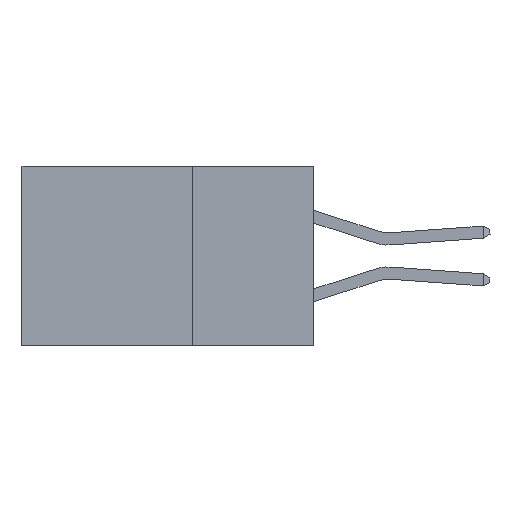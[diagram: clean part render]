
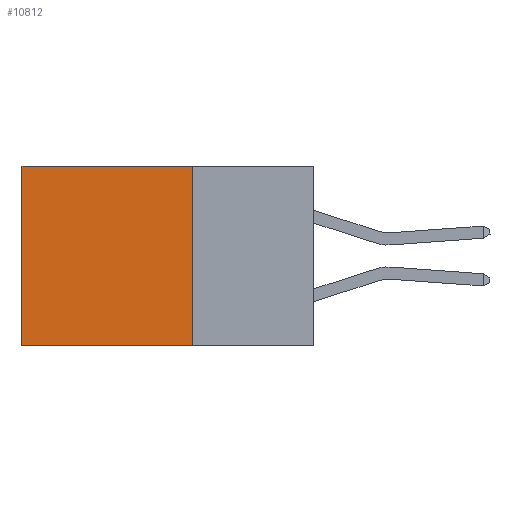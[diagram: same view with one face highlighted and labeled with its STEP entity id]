
A CAD part, left-side view. The second image highlights one B-rep face of the part: STEP entity #10812.
In plain terms, the highlighted planar face has unit normal (-1, 0, 0).
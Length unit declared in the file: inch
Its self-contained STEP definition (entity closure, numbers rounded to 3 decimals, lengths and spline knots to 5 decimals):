
#524 = VERTEX_POINT ( 'NONE', #8475 ) ;
#650 = CARTESIAN_POINT ( 'NONE',  ( 0.2875, 0.6, -0.37 ) ) ;
#736 = VERTEX_POINT ( 'NONE', #650 ) ;
#1175 = ORIENTED_EDGE ( 'NONE', *, *, #7287, .F. ) ;
#1316 = DIRECTION ( 'NONE',  ( 0., 0., -1. ) ) ;
#1529 = VERTEX_POINT ( 'NONE', #6416 ) ;
#2299 = FACE_OUTER_BOUND ( 'NONE', #17445, .T. ) ;
#2832 = CARTESIAN_POINT ( 'NONE',  ( 0.2875, 0.6, 0. ) ) ;
#3525 = CARTESIAN_POINT ( 'NONE',  ( 0.2875, 0.25, 0. ) ) ;
#3719 = EDGE_CURVE ( 'NONE', #524, #4255, #9459, .T. ) ;
#4255 = VERTEX_POINT ( 'NONE', #15955 ) ;
#4601 = CARTESIAN_POINT ( 'NONE',  ( 0.2875, 0.25, -0.37 ) ) ;
#4879 = VECTOR ( 'NONE', #18082, 39.37008 ) ;
#4885 = ORIENTED_EDGE ( 'NONE', *, *, #3719, .T. ) ;
#5474 = LINE ( 'NONE', #2832, #13375 ) ;
#6416 = CARTESIAN_POINT ( 'NONE',  ( 0.2875, 0.25, -0.37 ) ) ;
#6682 = LINE ( 'NONE', #12396, #4879 ) ;
#7287 = EDGE_CURVE ( 'NONE', #524, #1529, #6682, .T. ) ;
#7562 = DIRECTION ( 'NONE',  ( 0., 1., 0. ) ) ;
#7720 = ORIENTED_EDGE ( 'NONE', *, *, #15877, .F. ) ;
#8475 = CARTESIAN_POINT ( 'NONE',  ( 0.2875, 0.25, 0. ) ) ;
#9261 = DIRECTION ( 'NONE',  ( 1., 0., 0. ) ) ;
#9379 = ORIENTED_EDGE ( 'NONE', *, *, #12610, .T. ) ;
#9459 = LINE ( 'NONE', #9845, #10948 ) ;
#9845 = CARTESIAN_POINT ( 'NONE',  ( 0.2875, 0.25, 0. ) ) ;
#10771 = PLANE ( 'NONE',  #17186 ) ;
#10812 = ADVANCED_FACE ( 'NONE', ( #2299 ), #10771, .F. ) ;
#10948 = VECTOR ( 'NONE', #7562, 39.37008 ) ;
#12072 = DIRECTION ( 'NONE',  ( 0., 0., -1. ) ) ;
#12396 = CARTESIAN_POINT ( 'NONE',  ( 0.2875, 0.25, 0. ) ) ;
#12610 = EDGE_CURVE ( 'NONE', #4255, #736, #5474, .T. ) ;
#13159 = DIRECTION ( 'NONE',  ( 0., 1., 0. ) ) ;
#13375 = VECTOR ( 'NONE', #1316, 39.37008 ) ;
#14748 = LINE ( 'NONE', #4601, #18512 ) ;
#15877 = EDGE_CURVE ( 'NONE', #1529, #736, #14748, .T. ) ;
#15955 = CARTESIAN_POINT ( 'NONE',  ( 0.2875, 0.6, 0. ) ) ;
#17186 = AXIS2_PLACEMENT_3D ( 'NONE', #3525, #9261, #12072 ) ;
#17445 = EDGE_LOOP ( 'NONE', ( #9379, #7720, #1175, #4885 ) ) ;
#18082 = DIRECTION ( 'NONE',  ( 0., 0., -1. ) ) ;
#18512 = VECTOR ( 'NONE', #13159, 39.37008 ) ;
